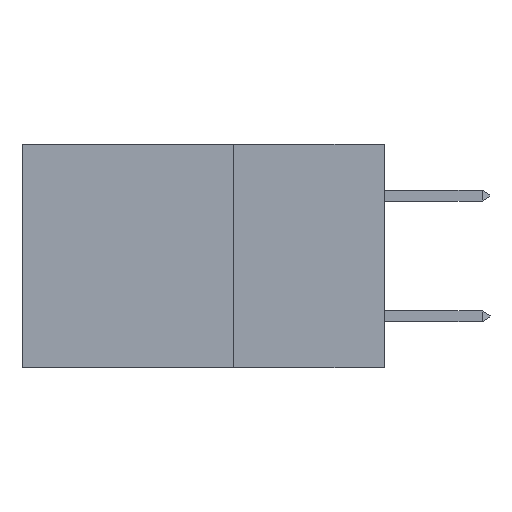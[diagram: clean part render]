
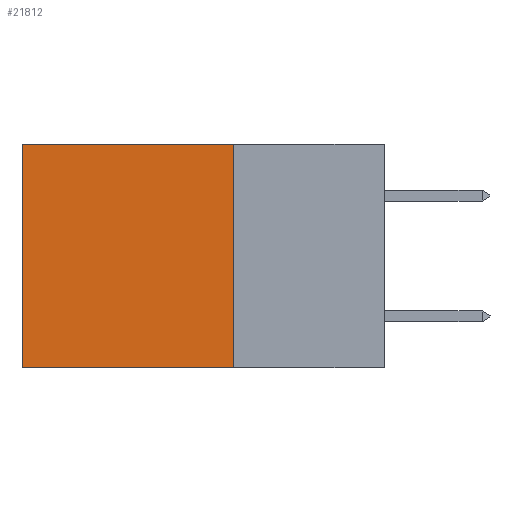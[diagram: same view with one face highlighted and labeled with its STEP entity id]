
A CAD part, left-side view. The second image highlights one B-rep face of the part: STEP entity #21812.
In plain terms, the highlighted planar face has unit normal (-1, 0, 0).
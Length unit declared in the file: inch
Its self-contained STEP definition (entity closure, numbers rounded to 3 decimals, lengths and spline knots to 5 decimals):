
#305 = CARTESIAN_POINT ( 'NONE',  ( 0.2875, 0.25, -0.37 ) ) ;
#2351 = DIRECTION ( 'NONE',  ( 0., 0., -1. ) ) ;
#2707 = LINE ( 'NONE', #305, #20088 ) ;
#3773 = VERTEX_POINT ( 'NONE', #29682 ) ;
#5173 = AXIS2_PLACEMENT_3D ( 'NONE', #28114, #11163, #20926 ) ;
#5481 = PLANE ( 'NONE',  #5173 ) ;
#5579 = EDGE_CURVE ( 'NONE', #16794, #3773, #19448, .T. ) ;
#5965 = ORIENTED_EDGE ( 'NONE', *, *, #5579, .F. ) ;
#6307 = CARTESIAN_POINT ( 'NONE',  ( 0.2875, 0.6, -0.37 ) ) ;
#6654 = CARTESIAN_POINT ( 'NONE',  ( 0.2875, 0.25, 0. ) ) ;
#6994 = ORIENTED_EDGE ( 'NONE', *, *, #7606, .T. ) ;
#7606 = EDGE_CURVE ( 'NONE', #16794, #19382, #14053, .T. ) ;
#9859 = VECTOR ( 'NONE', #2351, 39.37008 ) ;
#9879 = DIRECTION ( 'NONE',  ( 0., 1., 0. ) ) ;
#11163 = DIRECTION ( 'NONE',  ( 1., 0., 0. ) ) ;
#13566 = FACE_OUTER_BOUND ( 'NONE', #19505, .T. ) ;
#14053 = LINE ( 'NONE', #26368, #18181 ) ;
#16794 = VERTEX_POINT ( 'NONE', #6654 ) ;
#17975 = VECTOR ( 'NONE', #30483, 39.37008 ) ;
#18181 = VECTOR ( 'NONE', #23348, 39.37008 ) ;
#19382 = VERTEX_POINT ( 'NONE', #23793 ) ;
#19448 = LINE ( 'NONE', #19917, #9859 ) ;
#19505 = EDGE_LOOP ( 'NONE', ( #28251, #21859, #5965, #6994 ) ) ;
#19917 = CARTESIAN_POINT ( 'NONE',  ( 0.2875, 0.25, 0. ) ) ;
#20088 = VECTOR ( 'NONE', #9879, 39.37008 ) ;
#20737 = CARTESIAN_POINT ( 'NONE',  ( 0.2875, 0.6, 0. ) ) ;
#20926 = DIRECTION ( 'NONE',  ( 0., 0., -1. ) ) ;
#21812 = ADVANCED_FACE ( 'NONE', ( #13566 ), #5481, .F. ) ;
#21859 = ORIENTED_EDGE ( 'NONE', *, *, #27743, .F. ) ;
#23348 = DIRECTION ( 'NONE',  ( 0., 1., 0. ) ) ;
#23793 = CARTESIAN_POINT ( 'NONE',  ( 0.2875, 0.6, 0. ) ) ;
#25135 = VERTEX_POINT ( 'NONE', #6307 ) ;
#25694 = LINE ( 'NONE', #20737, #17975 ) ;
#25913 = EDGE_CURVE ( 'NONE', #19382, #25135, #25694, .T. ) ;
#26368 = CARTESIAN_POINT ( 'NONE',  ( 0.2875, 0.25, 0. ) ) ;
#27743 = EDGE_CURVE ( 'NONE', #3773, #25135, #2707, .T. ) ;
#28114 = CARTESIAN_POINT ( 'NONE',  ( 0.2875, 0.25, 0. ) ) ;
#28251 = ORIENTED_EDGE ( 'NONE', *, *, #25913, .T. ) ;
#29682 = CARTESIAN_POINT ( 'NONE',  ( 0.2875, 0.25, -0.37 ) ) ;
#30483 = DIRECTION ( 'NONE',  ( 0., 0., -1. ) ) ;
